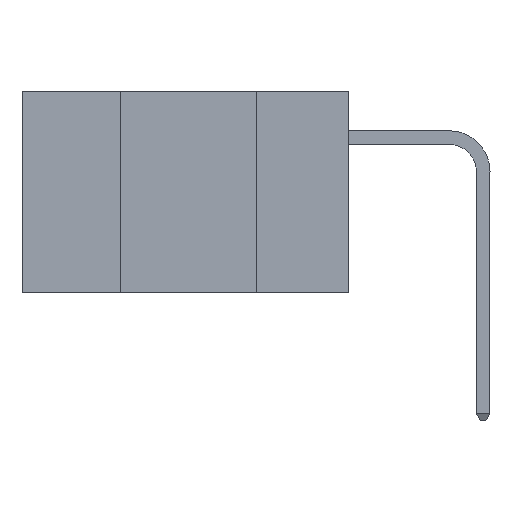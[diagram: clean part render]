
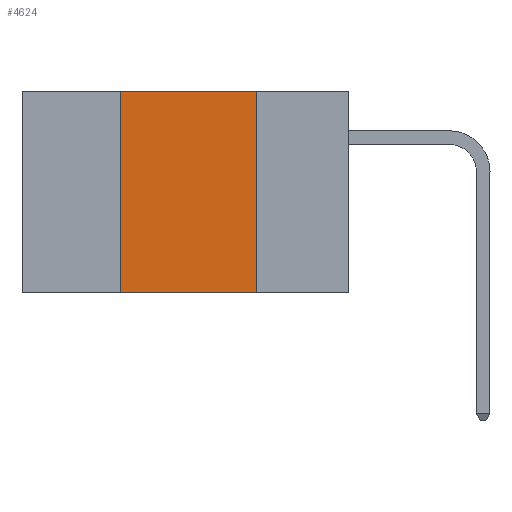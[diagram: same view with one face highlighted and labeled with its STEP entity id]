
A CAD part, left-side view. The second image highlights one B-rep face of the part: STEP entity #4624.
In plain terms, the highlighted planar face has unit normal (-1, 0, 0).
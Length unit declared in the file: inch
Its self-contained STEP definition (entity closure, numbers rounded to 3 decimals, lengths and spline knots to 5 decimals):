
#199 = CARTESIAN_POINT ( 'NONE',  ( 0., 0.6, 0. ) ) ;
#1022 = DIRECTION ( 'NONE',  ( 0., 0., -1. ) ) ;
#1200 = DIRECTION ( 'NONE',  ( 0., -1., 0. ) ) ;
#1398 = CARTESIAN_POINT ( 'NONE',  ( 0., 0.42, -0.37 ) ) ;
#1529 = LINE ( 'NONE', #11925, #11938 ) ;
#1541 = ORIENTED_EDGE ( 'NONE', *, *, #10112, .F. ) ;
#2918 = LINE ( 'NONE', #10742, #10775 ) ;
#3022 = CARTESIAN_POINT ( 'NONE',  ( 0., 0.17, 0. ) ) ;
#3147 = FACE_OUTER_BOUND ( 'NONE', #13848, .T. ) ;
#3388 = ORIENTED_EDGE ( 'NONE', *, *, #7206, .F. ) ;
#3768 = VECTOR ( 'NONE', #8917, 39.37008 ) ;
#3795 = AXIS2_PLACEMENT_3D ( 'NONE', #5605, #11991, #9794 ) ;
#4421 = EDGE_CURVE ( 'NONE', #9437, #7219, #8175, .T. ) ;
#4624 = ADVANCED_FACE ( 'NONE', ( #3147 ), #10829, .F. ) ;
#5605 = CARTESIAN_POINT ( 'NONE',  ( 0., 0.6, 0. ) ) ;
#6579 = LINE ( 'NONE', #199, #3768 ) ;
#6865 = CARTESIAN_POINT ( 'NONE',  ( 0., 0.17, -0.37 ) ) ;
#7206 = EDGE_CURVE ( 'NONE', #13898, #9313, #6579, .T. ) ;
#7219 = VERTEX_POINT ( 'NONE', #6865 ) ;
#7221 = CARTESIAN_POINT ( 'NONE',  ( 0., 0.42, 0. ) ) ;
#7473 = EDGE_CURVE ( 'NONE', #9437, #13898, #1529, .T. ) ;
#7675 = CARTESIAN_POINT ( 'NONE',  ( 0., 0.6, -0.37 ) ) ;
#8175 = LINE ( 'NONE', #7675, #13207 ) ;
#8909 = ORIENTED_EDGE ( 'NONE', *, *, #4421, .T. ) ;
#8917 = DIRECTION ( 'NONE',  ( 0., -1., 0. ) ) ;
#9313 = VERTEX_POINT ( 'NONE', #3022 ) ;
#9437 = VERTEX_POINT ( 'NONE', #1398 ) ;
#9794 = DIRECTION ( 'NONE',  ( 0., 0., -1. ) ) ;
#9922 = ORIENTED_EDGE ( 'NONE', *, *, #7473, .F. ) ;
#10112 = EDGE_CURVE ( 'NONE', #9313, #7219, #2918, .T. ) ;
#10742 = CARTESIAN_POINT ( 'NONE',  ( 0., 0.17, 0. ) ) ;
#10775 = VECTOR ( 'NONE', #1022, 39.37008 ) ;
#10829 = PLANE ( 'NONE',  #3795 ) ;
#11419 = DIRECTION ( 'NONE',  ( 0., 0., 1. ) ) ;
#11925 = CARTESIAN_POINT ( 'NONE',  ( 0., 0.42, 0. ) ) ;
#11938 = VECTOR ( 'NONE', #11419, 39.37008 ) ;
#11991 = DIRECTION ( 'NONE',  ( 1., 0., 0. ) ) ;
#13207 = VECTOR ( 'NONE', #1200, 39.37008 ) ;
#13848 = EDGE_LOOP ( 'NONE', ( #1541, #3388, #9922, #8909 ) ) ;
#13898 = VERTEX_POINT ( 'NONE', #7221 ) ;
